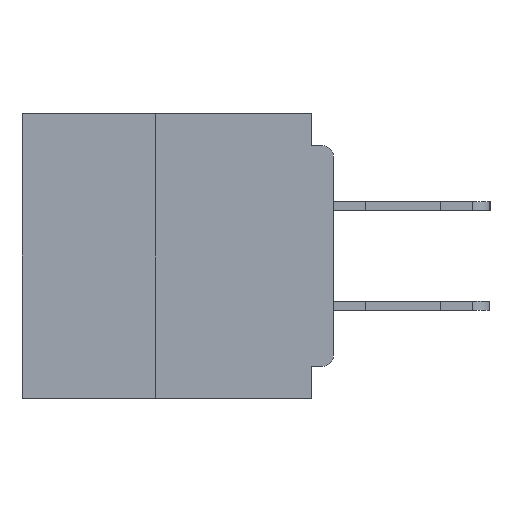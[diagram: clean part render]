
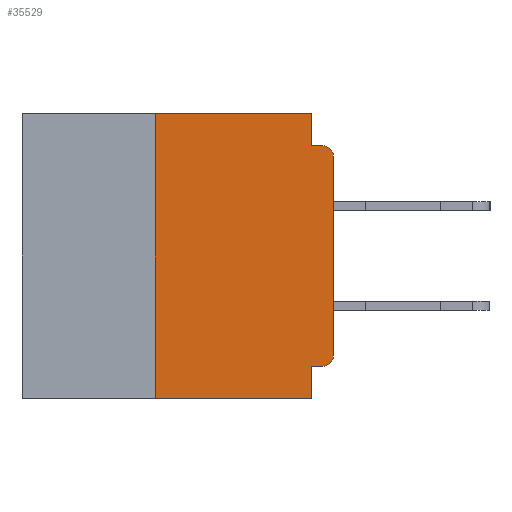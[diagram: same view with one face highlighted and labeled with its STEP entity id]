
A CAD part, left-side view. The second image highlights one B-rep face of the part: STEP entity #35529.
In plain terms, the highlighted planar face has unit normal (-1, 0, 0).
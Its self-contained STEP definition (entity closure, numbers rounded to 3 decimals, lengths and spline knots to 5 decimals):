
#580 = ORIENTED_EDGE ( 'NONE', *, *, #43144, .F. ) ;
#1596 = ORIENTED_EDGE ( 'NONE', *, *, #5971, .T. ) ;
#1598 = VERTEX_POINT ( 'NONE', #53172 ) ;
#1814 = LINE ( 'NONE', #2342, #23696 ) ;
#2342 = CARTESIAN_POINT ( 'NONE',  ( 0., 0., -0.045 ) ) ;
#2355 = DIRECTION ( 'NONE',  ( 0., 0., -1. ) ) ;
#2542 = DIRECTION ( 'NONE',  ( 0., -1., 0. ) ) ;
#3891 = ORIENTED_EDGE ( 'NONE', *, *, #15711, .T. ) ;
#3908 = AXIS2_PLACEMENT_3D ( 'NONE', #58430, #30427, #2355 ) ;
#4141 = CARTESIAN_POINT ( 'NONE',  ( 0., 0.437, 0. ) ) ;
#5971 = EDGE_CURVE ( 'NONE', #19340, #18857, #38677, .T. ) ;
#6565 = CARTESIAN_POINT ( 'NONE',  ( 0., 0.25, 0. ) ) ;
#6622 = ORIENTED_EDGE ( 'NONE', *, *, #47044, .F. ) ;
#6980 = VERTEX_POINT ( 'NONE', #42590 ) ;
#7457 = VECTOR ( 'NONE', #58214, 39.37008 ) ;
#8280 = VERTEX_POINT ( 'NONE', #57273 ) ;
#8736 = VERTEX_POINT ( 'NONE', #51501 ) ;
#11082 = CARTESIAN_POINT ( 'NONE',  ( 0., 0.031, 0. ) ) ;
#11331 = AXIS2_PLACEMENT_3D ( 'NONE', #14030, #46844, #18710 ) ;
#12717 = CARTESIAN_POINT ( 'NONE',  ( 0., 0.437, -0.4 ) ) ;
#13621 = DIRECTION ( 'NONE',  ( 0., 0., 1. ) ) ;
#13655 = CARTESIAN_POINT ( 'NONE',  ( 0., 0.031, -0.045 ) ) ;
#13747 = DIRECTION ( 'NONE',  ( 0., -1., 0. ) ) ;
#14030 = CARTESIAN_POINT ( 'NONE',  ( 0., 0.437, 0. ) ) ;
#15711 = EDGE_CURVE ( 'NONE', #17524, #1598, #22665, .T. ) ;
#16369 = CARTESIAN_POINT ( 'NONE',  ( 0., 0.015, -0.34 ) ) ;
#17383 = DIRECTION ( 'NONE',  ( 0., -1., 0. ) ) ;
#17524 = VERTEX_POINT ( 'NONE', #47563 ) ;
#17774 = LINE ( 'NONE', #11082, #42805 ) ;
#17879 = VECTOR ( 'NONE', #17383, 39.37008 ) ;
#18710 = DIRECTION ( 'NONE',  ( 0., 0., -1. ) ) ;
#18857 = VERTEX_POINT ( 'NONE', #38620 ) ;
#19320 = VECTOR ( 'NONE', #22011, 39.37008 ) ;
#19340 = VERTEX_POINT ( 'NONE', #47573 ) ;
#19885 = LINE ( 'NONE', #25425, #7457 ) ;
#21088 = DIRECTION ( 'NONE',  ( 0., 0., -1. ) ) ;
#22011 = DIRECTION ( 'NONE',  ( 0., 0., -1. ) ) ;
#22460 = LINE ( 'NONE', #24210, #44577 ) ;
#22665 = CIRCLE ( 'NONE', #42793, 0.015 ) ;
#23212 = PLANE ( 'NONE',  #11331 ) ;
#23332 = LINE ( 'NONE', #37002, #46870 ) ;
#23696 = VECTOR ( 'NONE', #2542, 39.37008 ) ;
#24210 = CARTESIAN_POINT ( 'NONE',  ( 0., 0., -0.355 ) ) ;
#25425 = CARTESIAN_POINT ( 'NONE',  ( 0., 0.25, -0.4 ) ) ;
#26352 = VERTEX_POINT ( 'NONE', #35442 ) ;
#27518 = ORIENTED_EDGE ( 'NONE', *, *, #31923, .T. ) ;
#30427 = DIRECTION ( 'NONE',  ( -1., 0., 0. ) ) ;
#31923 = EDGE_CURVE ( 'NONE', #6980, #8736, #42909, .T. ) ;
#33336 = LINE ( 'NONE', #54631, #19320 ) ;
#34671 = VERTEX_POINT ( 'NONE', #6565 ) ;
#35442 = CARTESIAN_POINT ( 'NONE',  ( 0., 0.031, -0.355 ) ) ;
#35529 = ADVANCED_FACE ( 'NONE', ( #47056 ), #23212, .F. ) ;
#35599 = ORIENTED_EDGE ( 'NONE', *, *, #48506, .T. ) ;
#36082 = VECTOR ( 'NONE', #13747, 39.37008 ) ;
#36875 = ORIENTED_EDGE ( 'NONE', *, *, #59034, .F. ) ;
#37002 = CARTESIAN_POINT ( 'NONE',  ( 0., 0., 0. ) ) ;
#38620 = CARTESIAN_POINT ( 'NONE',  ( 0., 0.015, -0.045 ) ) ;
#38677 = CIRCLE ( 'NONE', #3908, 0.015 ) ;
#41806 = EDGE_CURVE ( 'NONE', #45720, #18857, #1814, .T. ) ;
#42590 = CARTESIAN_POINT ( 'NONE',  ( 0., 0.25, -0.4 ) ) ;
#42793 = AXIS2_PLACEMENT_3D ( 'NONE', #16369, #49190, #21088 ) ;
#42805 = VECTOR ( 'NONE', #43932, 39.37008 ) ;
#42909 = LINE ( 'NONE', #12717, #17879 ) ;
#42957 = DIRECTION ( 'NONE',  ( 0., 1., 0. ) ) ;
#43089 = ORIENTED_EDGE ( 'NONE', *, *, #49603, .F. ) ;
#43144 = EDGE_CURVE ( 'NONE', #34671, #8280, #48532, .T. ) ;
#43932 = DIRECTION ( 'NONE',  ( 0., 0., -1. ) ) ;
#44577 = VECTOR ( 'NONE', #42957, 39.37008 ) ;
#45720 = VERTEX_POINT ( 'NONE', #13655 ) ;
#46844 = DIRECTION ( 'NONE',  ( 1., 0., 0. ) ) ;
#46870 = VECTOR ( 'NONE', #13621, 39.37008 ) ;
#47044 = EDGE_CURVE ( 'NONE', #6980, #34671, #19885, .T. ) ;
#47056 = FACE_OUTER_BOUND ( 'NONE', #55642, .T. ) ;
#47563 = CARTESIAN_POINT ( 'NONE',  ( 0., 0.015, -0.355 ) ) ;
#47573 = CARTESIAN_POINT ( 'NONE',  ( 0., 0., -0.06 ) ) ;
#48506 = EDGE_CURVE ( 'NONE', #1598, #19340, #23332, .T. ) ;
#48532 = LINE ( 'NONE', #4141, #36082 ) ;
#48547 = ORIENTED_EDGE ( 'NONE', *, *, #41806, .F. ) ;
#49190 = DIRECTION ( 'NONE',  ( -1., 0., 0. ) ) ;
#49603 = EDGE_CURVE ( 'NONE', #17524, #26352, #22460, .T. ) ;
#51501 = CARTESIAN_POINT ( 'NONE',  ( 0., 0.031, -0.4 ) ) ;
#52078 = EDGE_CURVE ( 'NONE', #26352, #8736, #33336, .T. ) ;
#53172 = CARTESIAN_POINT ( 'NONE',  ( 0., 0., -0.34 ) ) ;
#54631 = CARTESIAN_POINT ( 'NONE',  ( 0., 0.031, -0.4 ) ) ;
#55642 = EDGE_LOOP ( 'NONE', ( #35599, #1596, #48547, #36875, #580, #6622, #27518, #57910, #43089, #3891 ) ) ;
#57273 = CARTESIAN_POINT ( 'NONE',  ( 0., 0.031, 0. ) ) ;
#57910 = ORIENTED_EDGE ( 'NONE', *, *, #52078, .F. ) ;
#58214 = DIRECTION ( 'NONE',  ( 0., 0., 1. ) ) ;
#58430 = CARTESIAN_POINT ( 'NONE',  ( 0., 0.015, -0.06 ) ) ;
#59034 = EDGE_CURVE ( 'NONE', #8280, #45720, #17774, .T. ) ;
